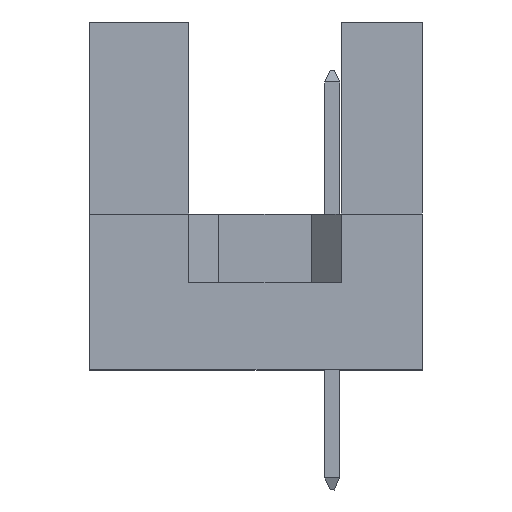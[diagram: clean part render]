
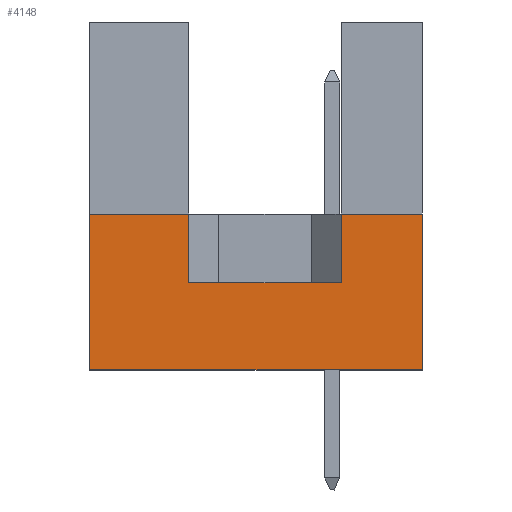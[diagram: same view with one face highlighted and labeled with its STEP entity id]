
A CAD part, left-side view. The second image highlights one B-rep face of the part: STEP entity #4148.
In plain terms, the highlighted planar face has unit normal (-1, 0, 0).
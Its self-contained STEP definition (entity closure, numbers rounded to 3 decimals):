
#370 = CARTESIAN_POINT ( 'NONE',  ( -47.5, 2.71, 2.9 ) ) ;
#420 = VECTOR ( 'NONE', #14210, 1000. ) ;
#426 = ORIENTED_EDGE ( 'NONE', *, *, #7507, .F. ) ;
#897 = DIRECTION ( 'NONE',  ( 0., 0., 1. ) ) ;
#1338 = CARTESIAN_POINT ( 'NONE',  ( -47.5, 7.79, 2.9 ) ) ;
#1441 = CARTESIAN_POINT ( 'NONE',  ( -47.5, 0., 0. ) ) ;
#1489 = EDGE_CURVE ( 'NONE', #8539, #4160, #7430, .T. ) ;
#1792 = ORIENTED_EDGE ( 'NONE', *, *, #11828, .T. ) ;
#2610 = FACE_OUTER_BOUND ( 'NONE', #6112, .T. ) ;
#2869 = AXIS2_PLACEMENT_3D ( 'NONE', #14724, #12476, #11098 ) ;
#2980 = LINE ( 'NONE', #13885, #7713 ) ;
#3371 = VECTOR ( 'NONE', #5102, 1000. ) ;
#3379 = EDGE_CURVE ( 'NONE', #14053, #8539, #2980, .T. ) ;
#3696 = VERTEX_POINT ( 'NONE', #6083 ) ;
#3916 = EDGE_CURVE ( 'NONE', #4160, #6143, #13120, .T. ) ;
#4148 = ADVANCED_FACE ( 'NONE', ( #2610 ), #7329, .F. ) ;
#4160 = VERTEX_POINT ( 'NONE', #5006 ) ;
#5006 = CARTESIAN_POINT ( 'NONE',  ( -47.5, 2.71, 5.2 ) ) ;
#5102 = DIRECTION ( 'NONE',  ( 0., 0., 1. ) ) ;
#5228 = CARTESIAN_POINT ( 'NONE',  ( -47.5, 11.1, 0. ) ) ;
#6064 = DIRECTION ( 'NONE',  ( 0., 0., 1. ) ) ;
#6083 = CARTESIAN_POINT ( 'NONE',  ( -47.5, 7.79, 5.2 ) ) ;
#6112 = EDGE_LOOP ( 'NONE', ( #13489, #1792, #426, #9637, #13174, #7030, #10203, #10877 ) ) ;
#6143 = VERTEX_POINT ( 'NONE', #7364 ) ;
#6476 = CARTESIAN_POINT ( 'NONE',  ( -47.5, 11.1, 0. ) ) ;
#6526 = EDGE_CURVE ( 'NONE', #6981, #6143, #7583, .T. ) ;
#6539 = CARTESIAN_POINT ( 'NONE',  ( -47.5, 2.71, 2.9 ) ) ;
#6981 = VERTEX_POINT ( 'NONE', #1441 ) ;
#7030 = ORIENTED_EDGE ( 'NONE', *, *, #6526, .T. ) ;
#7329 = PLANE ( 'NONE',  #2869 ) ;
#7364 = CARTESIAN_POINT ( 'NONE',  ( -47.5, 0., 5.2 ) ) ;
#7430 = LINE ( 'NONE', #6539, #3371 ) ;
#7507 = EDGE_CURVE ( 'NONE', #10537, #3696, #8019, .T. ) ;
#7583 = LINE ( 'NONE', #8709, #14484 ) ;
#7607 = CARTESIAN_POINT ( 'NONE',  ( -47.5, 7.79, 2.9 ) ) ;
#7713 = VECTOR ( 'NONE', #13744, 1000. ) ;
#7718 = LINE ( 'NONE', #1338, #12538 ) ;
#8019 = LINE ( 'NONE', #12923, #420 ) ;
#8134 = DIRECTION ( 'NONE',  ( 0., -1., 0. ) ) ;
#8170 = LINE ( 'NONE', #11872, #13842 ) ;
#8539 = VERTEX_POINT ( 'NONE', #370 ) ;
#8709 = CARTESIAN_POINT ( 'NONE',  ( -47.5, 0., 0. ) ) ;
#8918 = LINE ( 'NONE', #5228, #12865 ) ;
#9637 = ORIENTED_EDGE ( 'NONE', *, *, #12566, .F. ) ;
#10123 = DIRECTION ( 'NONE',  ( 0., 0., 1. ) ) ;
#10203 = ORIENTED_EDGE ( 'NONE', *, *, #3916, .F. ) ;
#10500 = VECTOR ( 'NONE', #8134, 1000. ) ;
#10537 = VERTEX_POINT ( 'NONE', #12692 ) ;
#10877 = ORIENTED_EDGE ( 'NONE', *, *, #1489, .F. ) ;
#11098 = DIRECTION ( 'NONE',  ( 0., 0., -1. ) ) ;
#11828 = EDGE_CURVE ( 'NONE', #14053, #3696, #7718, .T. ) ;
#11872 = CARTESIAN_POINT ( 'NONE',  ( -47.5, 11.1, 0. ) ) ;
#12476 = DIRECTION ( 'NONE',  ( 1., 0., 0. ) ) ;
#12538 = VECTOR ( 'NONE', #10123, 1000. ) ;
#12566 = EDGE_CURVE ( 'NONE', #14273, #10537, #8170, .T. ) ;
#12692 = CARTESIAN_POINT ( 'NONE',  ( -47.5, 11.1, 5.2 ) ) ;
#12865 = VECTOR ( 'NONE', #13820, 1000. ) ;
#12923 = CARTESIAN_POINT ( 'NONE',  ( -47.5, 11.1, 5.2 ) ) ;
#13120 = LINE ( 'NONE', #13199, #10500 ) ;
#13174 = ORIENTED_EDGE ( 'NONE', *, *, #15135, .T. ) ;
#13199 = CARTESIAN_POINT ( 'NONE',  ( -47.5, 11.1, 5.2 ) ) ;
#13489 = ORIENTED_EDGE ( 'NONE', *, *, #3379, .F. ) ;
#13744 = DIRECTION ( 'NONE',  ( 0., -1., 0. ) ) ;
#13820 = DIRECTION ( 'NONE',  ( 0., -1., 0. ) ) ;
#13842 = VECTOR ( 'NONE', #897, 1000. ) ;
#13885 = CARTESIAN_POINT ( 'NONE',  ( -47.5, 7.79, 2.9 ) ) ;
#14053 = VERTEX_POINT ( 'NONE', #7607 ) ;
#14210 = DIRECTION ( 'NONE',  ( 0., -1., 0. ) ) ;
#14273 = VERTEX_POINT ( 'NONE', #6476 ) ;
#14484 = VECTOR ( 'NONE', #6064, 1000. ) ;
#14724 = CARTESIAN_POINT ( 'NONE',  ( -47.5, 11.1, 0. ) ) ;
#15135 = EDGE_CURVE ( 'NONE', #14273, #6981, #8918, .T. ) ;
